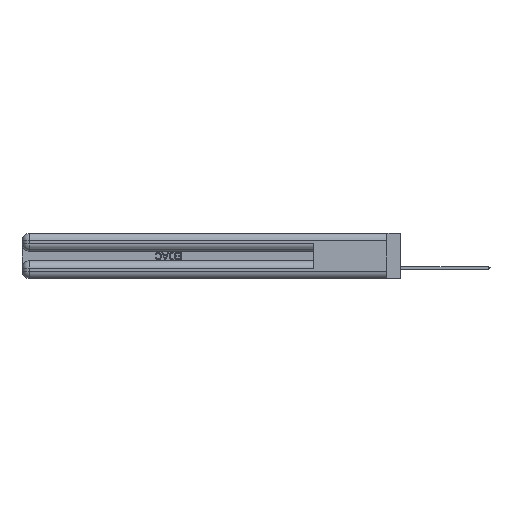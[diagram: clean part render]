
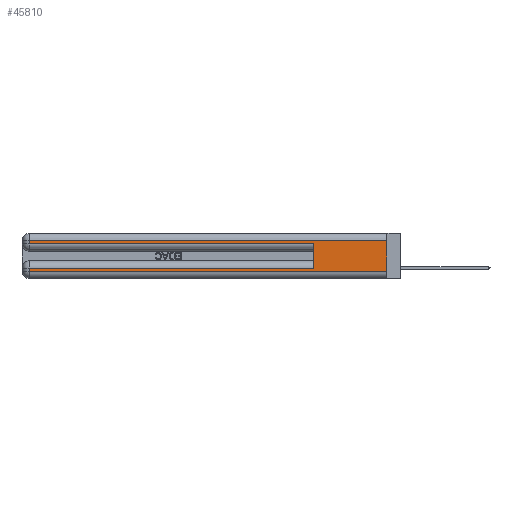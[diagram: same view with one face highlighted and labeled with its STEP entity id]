
A CAD part, left-side view. The second image highlights one B-rep face of the part: STEP entity #45810.
In plain terms, the highlighted planar face has unit normal (-1, 0, 0).
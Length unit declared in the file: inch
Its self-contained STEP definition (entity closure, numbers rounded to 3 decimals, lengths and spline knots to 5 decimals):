
#386 = LINE ( 'NONE', #46997, #15754 ) ;
#792 = VERTEX_POINT ( 'NONE', #44716 ) ;
#2254 = CARTESIAN_POINT ( 'NONE',  ( 0., 2.94, 0.06 ) ) ;
#2641 = EDGE_CURVE ( 'NONE', #13501, #47250, #9598, .T. ) ;
#3284 = VERTEX_POINT ( 'NONE', #31866 ) ;
#3903 = DIRECTION ( 'NONE',  ( 0., 0., -1. ) ) ;
#4994 = VERTEX_POINT ( 'NONE', #19767 ) ;
#5707 = DIRECTION ( 'NONE',  ( 0., 0., -1. ) ) ;
#6527 = ORIENTED_EDGE ( 'NONE', *, *, #27061, .T. ) ;
#6534 = CARTESIAN_POINT ( 'NONE',  ( 0., 2.94, 0.31 ) ) ;
#7526 = LINE ( 'NONE', #15274, #23524 ) ;
#8639 = LINE ( 'NONE', #25951, #11672 ) ;
#9393 = ORIENTED_EDGE ( 'NONE', *, *, #34437, .T. ) ;
#9598 = LINE ( 'NONE', #19105, #37065 ) ;
#9869 = VECTOR ( 'NONE', #46308, 39.37008 ) ;
#9909 = CARTESIAN_POINT ( 'NONE',  ( 0., 0., 0.06 ) ) ;
#10163 = VECTOR ( 'NONE', #17268, 39.37008 ) ;
#10211 = PLANE ( 'NONE',  #47005 ) ;
#10545 = CARTESIAN_POINT ( 'NONE',  ( 0., 0., 0.37 ) ) ;
#11672 = VECTOR ( 'NONE', #34535, 39.37008 ) ;
#12144 = ORIENTED_EDGE ( 'NONE', *, *, #22144, .T. ) ;
#13501 = VERTEX_POINT ( 'NONE', #2254 ) ;
#13779 = VERTEX_POINT ( 'NONE', #27353 ) ;
#14062 = EDGE_LOOP ( 'NONE', ( #24353, #20651, #40266, #12144, #41139, #9393, #6527, #23076 ) ) ;
#15161 = CARTESIAN_POINT ( 'NONE',  ( 0., 2.94, 0.37 ) ) ;
#15274 = CARTESIAN_POINT ( 'NONE',  ( 0., 0., 0.085 ) ) ;
#15754 = VECTOR ( 'NONE', #24417, 39.37008 ) ;
#17268 = DIRECTION ( 'NONE',  ( 0., 1., 0. ) ) ;
#19101 = EDGE_CURVE ( 'NONE', #34880, #792, #24354, .T. ) ;
#19105 = CARTESIAN_POINT ( 'NONE',  ( 0., 0., 0.06 ) ) ;
#19767 = CARTESIAN_POINT ( 'NONE',  ( 0., 0.6, 0.285 ) ) ;
#20651 = ORIENTED_EDGE ( 'NONE', *, *, #40372, .T. ) ;
#20945 = CARTESIAN_POINT ( 'NONE',  ( 0., 0., 0.37 ) ) ;
#21217 = DIRECTION ( 'NONE',  ( 1., 0., 0. ) ) ;
#21541 = DIRECTION ( 'NONE',  ( 0., 0., -1. ) ) ;
#21793 = EDGE_CURVE ( 'NONE', #13779, #4994, #8639, .T. ) ;
#22144 = EDGE_CURVE ( 'NONE', #792, #4994, #386, .T. ) ;
#23076 = ORIENTED_EDGE ( 'NONE', *, *, #2641, .T. ) ;
#23524 = VECTOR ( 'NONE', #34378, 39.37008 ) ;
#24353 = ORIENTED_EDGE ( 'NONE', *, *, #34728, .F. ) ;
#24354 = LINE ( 'NONE', #15161, #29163 ) ;
#24417 = DIRECTION ( 'NONE',  ( 0., -1., 0. ) ) ;
#25951 = CARTESIAN_POINT ( 'NONE',  ( 0., 0.6, 0.145 ) ) ;
#27061 = EDGE_CURVE ( 'NONE', #3284, #13501, #48494, .T. ) ;
#27353 = CARTESIAN_POINT ( 'NONE',  ( 0., 0.6, 0.085 ) ) ;
#28363 = CARTESIAN_POINT ( 'NONE',  ( 0., 0., 0.31 ) ) ;
#29163 = VECTOR ( 'NONE', #3903, 39.37008 ) ;
#31866 = CARTESIAN_POINT ( 'NONE',  ( 0., 2.94, 0.085 ) ) ;
#32110 = LINE ( 'NONE', #36250, #10163 ) ;
#34378 = DIRECTION ( 'NONE',  ( 0., 1., 0. ) ) ;
#34437 = EDGE_CURVE ( 'NONE', #13779, #3284, #7526, .T. ) ;
#34535 = DIRECTION ( 'NONE',  ( 0., 0., 1. ) ) ;
#34728 = EDGE_CURVE ( 'NONE', #34804, #47250, #34781, .T. ) ;
#34781 = LINE ( 'NONE', #20945, #46663 ) ;
#34804 = VERTEX_POINT ( 'NONE', #28363 ) ;
#34880 = VERTEX_POINT ( 'NONE', #6534 ) ;
#36250 = CARTESIAN_POINT ( 'NONE',  ( 0., 0., 0.31 ) ) ;
#37065 = VECTOR ( 'NONE', #48615, 39.37008 ) ;
#38850 = CARTESIAN_POINT ( 'NONE',  ( 0., 2.94, 0.37 ) ) ;
#40266 = ORIENTED_EDGE ( 'NONE', *, *, #19101, .T. ) ;
#40372 = EDGE_CURVE ( 'NONE', #34804, #34880, #32110, .T. ) ;
#41139 = ORIENTED_EDGE ( 'NONE', *, *, #21793, .F. ) ;
#43630 = FACE_OUTER_BOUND ( 'NONE', #14062, .T. ) ;
#44716 = CARTESIAN_POINT ( 'NONE',  ( 0., 2.94, 0.285 ) ) ;
#45810 = ADVANCED_FACE ( 'NONE', ( #43630 ), #10211, .F. ) ;
#46308 = DIRECTION ( 'NONE',  ( 0., 0., -1. ) ) ;
#46663 = VECTOR ( 'NONE', #5707, 39.37008 ) ;
#46997 = CARTESIAN_POINT ( 'NONE',  ( 0., 0., 0.285 ) ) ;
#47005 = AXIS2_PLACEMENT_3D ( 'NONE', #10545, #21217, #21541 ) ;
#47250 = VERTEX_POINT ( 'NONE', #9909 ) ;
#48494 = LINE ( 'NONE', #38850, #9869 ) ;
#48615 = DIRECTION ( 'NONE',  ( 0., -1., 0. ) ) ;
